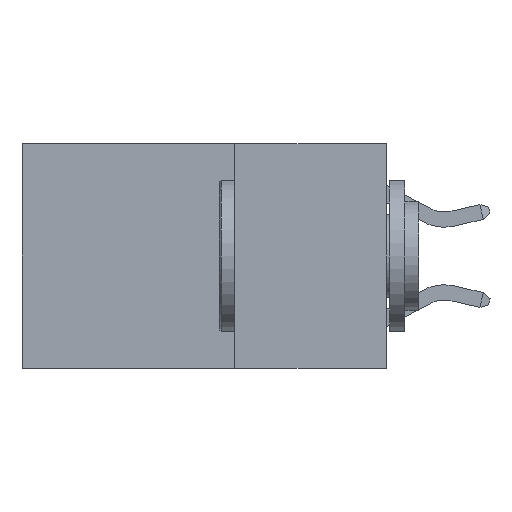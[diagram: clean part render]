
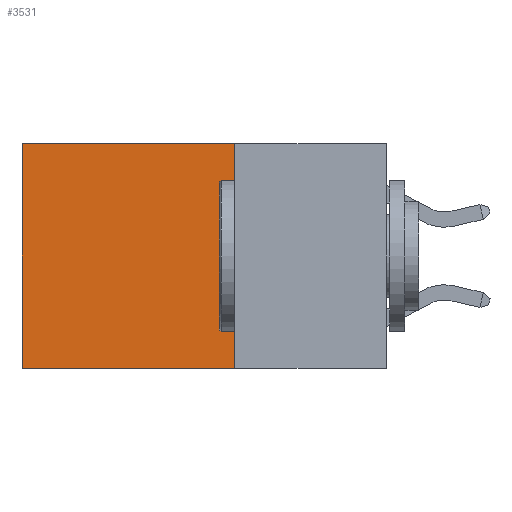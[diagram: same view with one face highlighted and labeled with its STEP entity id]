
A CAD part, left-side view. The second image highlights one B-rep face of the part: STEP entity #3531.
In plain terms, the highlighted planar face has unit normal (-1, 0, 0).
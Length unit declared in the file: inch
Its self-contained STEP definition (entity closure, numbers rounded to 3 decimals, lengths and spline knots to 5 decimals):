
#437 = EDGE_CURVE ( 'NONE', #19464, #957, #20065, .T. ) ;
#957 = VERTEX_POINT ( 'NONE', #19033 ) ;
#1342 = CARTESIAN_POINT ( 'NONE',  ( 0.2625, 0.25, 0. ) ) ;
#2503 = DIRECTION ( 'NONE',  ( 1., 0., 0. ) ) ;
#3531 = ADVANCED_FACE ( 'NONE', ( #9389 ), #12261, .F. ) ;
#3566 = VERTEX_POINT ( 'NONE', #9181 ) ;
#4124 = EDGE_LOOP ( 'NONE', ( #8186, #4435, #7582, #6637 ) ) ;
#4183 = DIRECTION ( 'NONE',  ( 0., 1., 0. ) ) ;
#4435 = ORIENTED_EDGE ( 'NONE', *, *, #437, .F. ) ;
#4578 = VECTOR ( 'NONE', #16474, 39.37008 ) ;
#5330 = LINE ( 'NONE', #16334, #12281 ) ;
#5789 = CARTESIAN_POINT ( 'NONE',  ( 0.2625, 0.25, 0. ) ) ;
#6637 = ORIENTED_EDGE ( 'NONE', *, *, #17539, .T. ) ;
#6914 = DIRECTION ( 'NONE',  ( 0., 0., -1. ) ) ;
#7582 = ORIENTED_EDGE ( 'NONE', *, *, #8721, .F. ) ;
#8186 = ORIENTED_EDGE ( 'NONE', *, *, #11975, .T. ) ;
#8487 = VECTOR ( 'NONE', #15484, 39.37008 ) ;
#8721 = EDGE_CURVE ( 'NONE', #15425, #19464, #20102, .T. ) ;
#9181 = CARTESIAN_POINT ( 'NONE',  ( 0.2625, 0.6, 0. ) ) ;
#9389 = FACE_OUTER_BOUND ( 'NONE', #4124, .T. ) ;
#10158 = VECTOR ( 'NONE', #4183, 39.37008 ) ;
#11975 = EDGE_CURVE ( 'NONE', #3566, #957, #5330, .T. ) ;
#12261 = PLANE ( 'NONE',  #20197 ) ;
#12281 = VECTOR ( 'NONE', #6914, 39.37008 ) ;
#13403 = CARTESIAN_POINT ( 'NONE',  ( 0.2625, 0.25, 0. ) ) ;
#13849 = LINE ( 'NONE', #5789, #10158 ) ;
#14343 = CARTESIAN_POINT ( 'NONE',  ( 0.2625, 0.25, -0.37 ) ) ;
#15425 = VERTEX_POINT ( 'NONE', #15792 ) ;
#15484 = DIRECTION ( 'NONE',  ( 0., 1., 0. ) ) ;
#15792 = CARTESIAN_POINT ( 'NONE',  ( 0.2625, 0.25, 0. ) ) ;
#16334 = CARTESIAN_POINT ( 'NONE',  ( 0.2625, 0.6, 0. ) ) ;
#16474 = DIRECTION ( 'NONE',  ( 0., 0., -1. ) ) ;
#16853 = CARTESIAN_POINT ( 'NONE',  ( 0.2625, 0.25, -0.37 ) ) ;
#17539 = EDGE_CURVE ( 'NONE', #15425, #3566, #13849, .T. ) ;
#19033 = CARTESIAN_POINT ( 'NONE',  ( 0.2625, 0.6, -0.37 ) ) ;
#19464 = VERTEX_POINT ( 'NONE', #14343 ) ;
#20065 = LINE ( 'NONE', #16853, #8487 ) ;
#20102 = LINE ( 'NONE', #13403, #4578 ) ;
#20197 = AXIS2_PLACEMENT_3D ( 'NONE', #1342, #2503, #20234 ) ;
#20234 = DIRECTION ( 'NONE',  ( 0., 0., -1. ) ) ;
